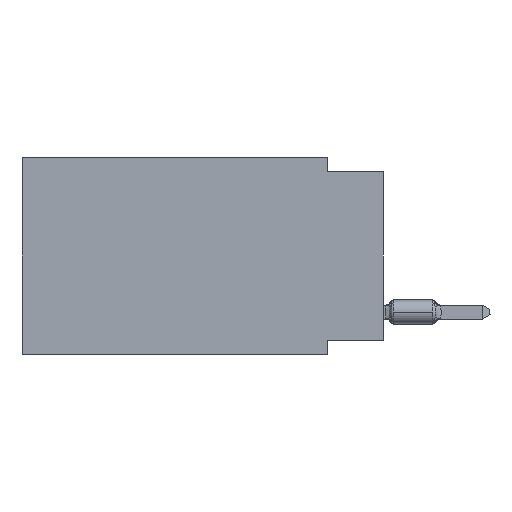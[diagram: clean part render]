
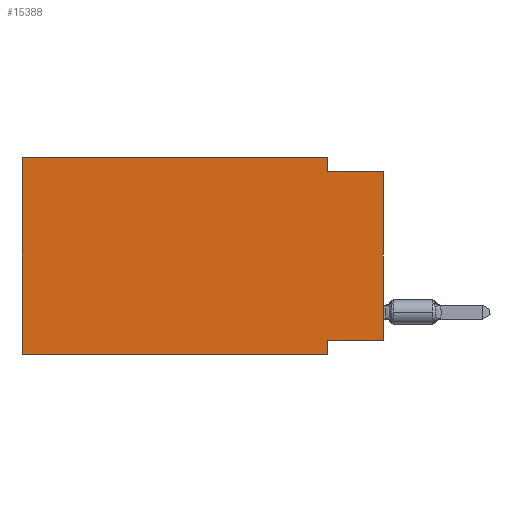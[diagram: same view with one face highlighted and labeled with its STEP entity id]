
A CAD part, left-side view. The second image highlights one B-rep face of the part: STEP entity #15388.
In plain terms, the highlighted planar face has unit normal (-1, 0, 0).
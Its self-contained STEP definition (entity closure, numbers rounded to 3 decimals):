
#1455 = ORIENTED_EDGE ( 'NONE', *, *, #16996, .F. ) ;
#1686 = CARTESIAN_POINT ( 'NONE',  ( 0., 16.383, 0. ) ) ;
#1697 = CARTESIAN_POINT ( 'NONE',  ( 0., 16.383, 0. ) ) ;
#2898 = CARTESIAN_POINT ( 'NONE',  ( 0., 2.54, -8.89 ) ) ;
#3558 = DIRECTION ( 'NONE',  ( 0., 1., 0. ) ) ;
#4298 = VERTEX_POINT ( 'NONE', #13600 ) ;
#5077 = ORIENTED_EDGE ( 'NONE', *, *, #12286, .F. ) ;
#6793 = ORIENTED_EDGE ( 'NONE', *, *, #28155, .F. ) ;
#7218 = VERTEX_POINT ( 'NONE', #41769 ) ;
#7567 = LINE ( 'NONE', #20986, #10984 ) ;
#7862 = LINE ( 'NONE', #1697, #33920 ) ;
#8208 = EDGE_CURVE ( 'NONE', #30989, #4298, #13651, .T. ) ;
#9176 = FACE_OUTER_BOUND ( 'NONE', #24907, .T. ) ;
#10039 = AXIS2_PLACEMENT_3D ( 'NONE', #36925, #20754, #27545 ) ;
#10984 = VECTOR ( 'NONE', #20572, 1000. ) ;
#11866 = CARTESIAN_POINT ( 'NONE',  ( 0., 2.54, -8.255 ) ) ;
#12286 = EDGE_CURVE ( 'NONE', #16791, #23295, #7862, .T. ) ;
#13600 = CARTESIAN_POINT ( 'NONE',  ( 0., 0., -0.635 ) ) ;
#13651 = LINE ( 'NONE', #39917, #37827 ) ;
#14026 = ORIENTED_EDGE ( 'NONE', *, *, #15068, .T. ) ;
#15068 = EDGE_CURVE ( 'NONE', #16791, #7218, #26455, .T. ) ;
#15259 = CARTESIAN_POINT ( 'NONE',  ( 0., 0., 0. ) ) ;
#15388 = ADVANCED_FACE ( 'NONE', ( #9176 ), #20124, .F. ) ;
#16009 = ORIENTED_EDGE ( 'NONE', *, *, #41468, .T. ) ;
#16533 = VECTOR ( 'NONE', #38436, 1000. ) ;
#16791 = VERTEX_POINT ( 'NONE', #32977 ) ;
#16996 = EDGE_CURVE ( 'NONE', #23295, #26828, #40014, .T. ) ;
#17391 = CARTESIAN_POINT ( 'NONE',  ( 0., 0., -8.255 ) ) ;
#18185 = ORIENTED_EDGE ( 'NONE', *, *, #8208, .F. ) ;
#20058 = ORIENTED_EDGE ( 'NONE', *, *, #36632, .F. ) ;
#20124 = PLANE ( 'NONE',  #10039 ) ;
#20572 = DIRECTION ( 'NONE',  ( 0., 0., -1. ) ) ;
#20754 = DIRECTION ( 'NONE',  ( 1., 0., 0. ) ) ;
#20986 = CARTESIAN_POINT ( 'NONE',  ( 0., 2.54, 0. ) ) ;
#21382 = EDGE_CURVE ( 'NONE', #29218, #41158, #39534, .T. ) ;
#23295 = VERTEX_POINT ( 'NONE', #36756 ) ;
#23626 = VECTOR ( 'NONE', #32843, 1000. ) ;
#23763 = ORIENTED_EDGE ( 'NONE', *, *, #21382, .F. ) ;
#24362 = CARTESIAN_POINT ( 'NONE',  ( 0., 0., -8.255 ) ) ;
#24907 = EDGE_LOOP ( 'NONE', ( #16009, #18185, #6793, #1455, #5077, #14026, #20058, #23763 ) ) ;
#26455 = LINE ( 'NONE', #35817, #23626 ) ;
#26725 = DIRECTION ( 'NONE',  ( 0., -1., 0. ) ) ;
#26828 = VERTEX_POINT ( 'NONE', #29689 ) ;
#27252 = DIRECTION ( 'NONE',  ( 0., 0., 1. ) ) ;
#27545 = DIRECTION ( 'NONE',  ( 0., 0., -1. ) ) ;
#27598 = CARTESIAN_POINT ( 'NONE',  ( 0., 2.54, -0.635 ) ) ;
#27797 = LINE ( 'NONE', #15259, #32832 ) ;
#28155 = EDGE_CURVE ( 'NONE', #26828, #30989, #7567, .T. ) ;
#29027 = VECTOR ( 'NONE', #40232, 1000. ) ;
#29218 = VERTEX_POINT ( 'NONE', #24362 ) ;
#29689 = CARTESIAN_POINT ( 'NONE',  ( 0., 2.54, 0. ) ) ;
#30989 = VERTEX_POINT ( 'NONE', #27598 ) ;
#31211 = LINE ( 'NONE', #2898, #16533 ) ;
#31816 = DIRECTION ( 'NONE',  ( 0., 0., 1. ) ) ;
#32832 = VECTOR ( 'NONE', #31816, 1000. ) ;
#32843 = DIRECTION ( 'NONE',  ( 0., -1., 0. ) ) ;
#32977 = CARTESIAN_POINT ( 'NONE',  ( 0., 16.383, -8.89 ) ) ;
#33920 = VECTOR ( 'NONE', #27252, 1000. ) ;
#35817 = CARTESIAN_POINT ( 'NONE',  ( 0., 16.383, -8.89 ) ) ;
#36632 = EDGE_CURVE ( 'NONE', #41158, #7218, #31211, .T. ) ;
#36756 = CARTESIAN_POINT ( 'NONE',  ( 0., 16.383, 0. ) ) ;
#36925 = CARTESIAN_POINT ( 'NONE',  ( 0., 16.383, 0. ) ) ;
#37827 = VECTOR ( 'NONE', #26725, 1000. ) ;
#38436 = DIRECTION ( 'NONE',  ( 0., 0., -1. ) ) ;
#39534 = LINE ( 'NONE', #17391, #40592 ) ;
#39917 = CARTESIAN_POINT ( 'NONE',  ( 0., 0., -0.635 ) ) ;
#40014 = LINE ( 'NONE', #1686, #29027 ) ;
#40232 = DIRECTION ( 'NONE',  ( 0., -1., 0. ) ) ;
#40592 = VECTOR ( 'NONE', #3558, 1000. ) ;
#41158 = VERTEX_POINT ( 'NONE', #11866 ) ;
#41468 = EDGE_CURVE ( 'NONE', #29218, #4298, #27797, .T. ) ;
#41769 = CARTESIAN_POINT ( 'NONE',  ( 0., 2.54, -8.89 ) ) ;
